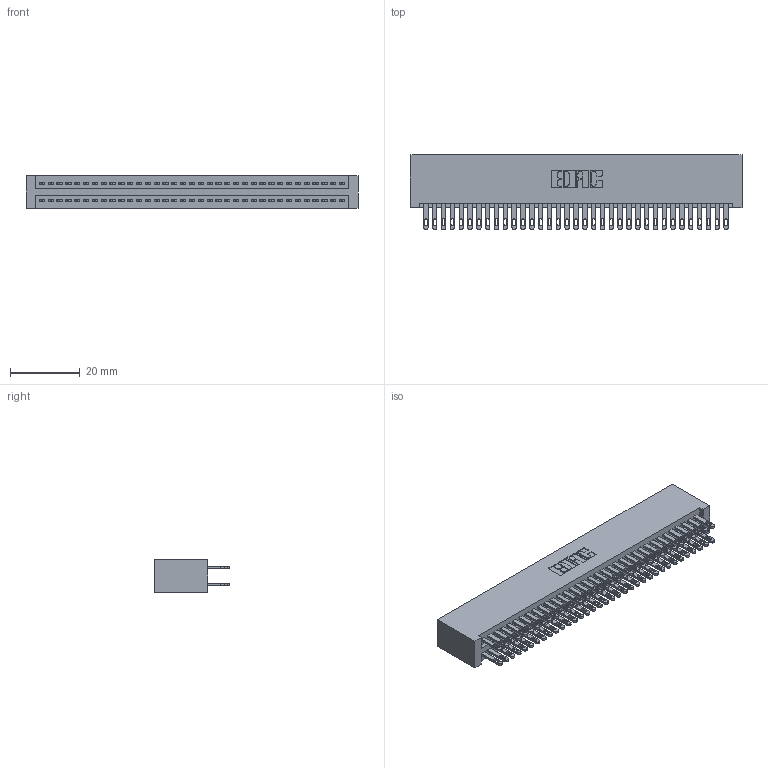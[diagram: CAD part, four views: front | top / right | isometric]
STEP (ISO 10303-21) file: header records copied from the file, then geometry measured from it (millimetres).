
FILE_DESCRIPTION (( 'STEP AP203' ), '1' );
FILE_NAME ('345-070-500-201.STEP', '2019-10-30T23:26:31', ( '' ), ( '' ), 'SwSTEP 2.0', 'SolidWorks 2016', '' );
FILE_SCHEMA (( 'CONFIG_CONTROL_DESIGN' ));
Length unit declared in the file: inch
Products named in the file (3): 345-292-001_345-293-100; 345 Part_No Mounting Lugs; 345-070-500-201
Assembly tree (71 placements, depth 2):
  345-070-500-201
    345 Part_No Mounting Lugs
    345-292-001_345-293-100  x70
Bounding box: 95.5 x 21.51 x 9.4 mm (x, y, z)
Volume: 10042.2 mm3; surface area: 15725.7 mm2
Topology: 71 solids, 71 shells, 3338 faces, 10187 edges, 6790 vertices
Faces by surface type: plane 1966, cylinder 1372
Entity records: 28057 total; most frequent: CARTESIAN_POINT 4708, ORIENTED_EDGE 4642, DIRECTION 4157, EDGE_CURVE 2321, LINE 2053, VECTOR 2053, VERTEX_POINT 1546, AXIS2_PLACEMENT_3D 1052
